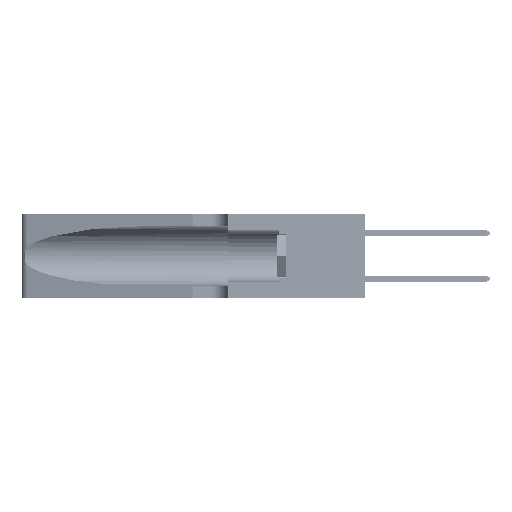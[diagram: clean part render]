
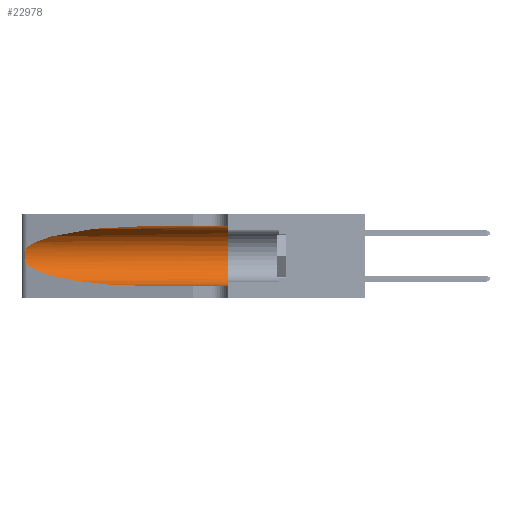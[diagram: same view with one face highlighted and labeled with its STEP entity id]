
A CAD part, left-side view. The second image highlights one B-rep face of the part: STEP entity #22978.
In plain terms, the highlighted cylindrical face has radius 3.308 mm (diameter 6.617 mm), a partial arc.
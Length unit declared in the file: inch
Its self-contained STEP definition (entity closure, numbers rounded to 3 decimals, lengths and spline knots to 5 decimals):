
#62 = CARTESIAN_POINT ( 'NONE',  ( 0.18966, 0.96281, 0.31525 ) ) ;
#373 =( BOUNDED_CURVE ( )  B_SPLINE_CURVE ( 3, ( #7837, #62, #42143, #19459 ),
 .UNSPECIFIED., .F., .F. ) 
 B_SPLINE_CURVE_WITH_KNOTS ( ( 4, 4 ),
 ( 1.5708, 2.84003 ),
 .UNSPECIFIED. ) 
 CURVE ( )  GEOMETRIC_REPRESENTATION_ITEM ( )  RATIONAL_B_SPLINE_CURVE ( ( 1., 0.87, 0.87, 1. ) ) 
 REPRESENTATION_ITEM ( '' )  );
#442 = ORIENTED_EDGE ( 'NONE', *, *, #43985, .F. ) ;
#2747 = CARTESIAN_POINT ( 'NONE',  ( 0.1305, 1.61858, 0.31525 ) ) ;
#2788 = CARTESIAN_POINT ( 'NONE',  ( 0.25487, 1.22718, 0.22369 ) ) ;
#5811 = ORIENTED_EDGE ( 'NONE', *, *, #29733, .F. ) ;
#6112 = DIRECTION ( 'NONE',  ( 0., 1., 0. ) ) ;
#6242 = VERTEX_POINT ( 'NONE', #46862 ) ;
#6470 = AXIS2_PLACEMENT_3D ( 'NONE', #29033, #6112, #32855 ) ;
#6654 = CARTESIAN_POINT ( 'NONE',  ( 0.25787, 1.23484, 0.2124 ) ) ;
#7378 = CYLINDRICAL_SURFACE ( 'NONE', #45912, 0.13025 ) ;
#7679 = LINE ( 'NONE', #2747, #47015 ) ;
#7837 = CARTESIAN_POINT ( 'NONE',  ( 0.1305, 0.72297, 0.31525 ) ) ;
#8088 = ORIENTED_EDGE ( 'NONE', *, *, #19232, .T. ) ;
#9329 = B_SPLINE_CURVE_WITH_KNOTS ( 'NONE', 3,
 ( #2788, #18099, #40841, #6654, #33392, #10520, #37198, #14399, #41004, #18273, #44805, #22125, #48634, #25943 ),
 .UNSPECIFIED., .F., .F.,
 ( 4, 2, 2, 2, 2, 2, 4 ),
 ( 0., 0.00027, 0.00053, 0.00107, 0.0016, 0.00187, 0.00214 ),
 .UNSPECIFIED. ) ;
#10520 = CARTESIAN_POINT ( 'NONE',  ( 0.26018, 1.23835, 0.19895 ) ) ;
#11185 = CARTESIAN_POINT ( 'NONE',  ( 0.18966, 0.96281, 0.05475 ) ) ;
#11971 = VERTEX_POINT ( 'NONE', #47407 ) ;
#13520 = ORIENTED_EDGE ( 'NONE', *, *, #34478, .T. ) ;
#14399 = CARTESIAN_POINT ( 'NONE',  ( 0.26075, 1.23896, 0.178 ) ) ;
#14514 = CARTESIAN_POINT ( 'NONE',  ( 0.25487, 1.22718, 0.14631 ) ) ;
#14601 =( BOUNDED_CURVE ( )  B_SPLINE_CURVE ( 3, ( #30231, #18780, #11185, #37859 ),
 .UNSPECIFIED., .F., .T. ) 
 B_SPLINE_CURVE_WITH_KNOTS ( ( 4, 4 ),
 ( 3.44316, 4.71239 ),
 .UNSPECIFIED. ) 
 CURVE ( )  GEOMETRIC_REPRESENTATION_ITEM ( )  RATIONAL_B_SPLINE_CURVE ( ( 1., 0.87, 0.87, 1. ) ) 
 REPRESENTATION_ITEM ( '' )  );
#16672 = CARTESIAN_POINT ( 'NONE',  ( 0.1305, 0.35, 0.31525 ) ) ;
#17841 = VERTEX_POINT ( 'NONE', #48037 ) ;
#18099 = CARTESIAN_POINT ( 'NONE',  ( 0.25555, 1.22994, 0.2215 ) ) ;
#18226 = DIRECTION ( 'NONE',  ( 0., -1., 0. ) ) ;
#18273 = CARTESIAN_POINT ( 'NONE',  ( 0.25856, 1.23593, 0.16098 ) ) ;
#18780 = CARTESIAN_POINT ( 'NONE',  ( 0.2373, 1.15595, 0.08982 ) ) ;
#19232 = EDGE_CURVE ( 'NONE', #17841, #11971, #25170, .T. ) ;
#19459 = CARTESIAN_POINT ( 'NONE',  ( 0.25487, 1.22718, 0.22369 ) ) ;
#21739 = CARTESIAN_POINT ( 'NONE',  ( 0.1305, 1.61858, 0.05475 ) ) ;
#22125 = CARTESIAN_POINT ( 'NONE',  ( 0.25639, 1.23186, 0.15144 ) ) ;
#22978 = ADVANCED_FACE ( 'NONE', ( #49098 ), #7378, .F. ) ;
#25170 = LINE ( 'NONE', #21739, #44121 ) ;
#25538 = DIRECTION ( 'NONE',  ( 0., -1., 0. ) ) ;
#25943 = CARTESIAN_POINT ( 'NONE',  ( 0.25487, 1.22718, 0.14631 ) ) ;
#29033 = CARTESIAN_POINT ( 'NONE',  ( 0.1305, 0.35, 0.185 ) ) ;
#29733 = EDGE_CURVE ( 'NONE', #42022, #11971, #30964, .T. ) ;
#30231 = CARTESIAN_POINT ( 'NONE',  ( 0.25487, 1.22718, 0.14631 ) ) ;
#30964 = CIRCLE ( 'NONE', #6470, 0.13025 ) ;
#31863 = CARTESIAN_POINT ( 'NONE',  ( 0.1305, 1.61858, 0.185 ) ) ;
#32312 = EDGE_CURVE ( 'NONE', #39011, #35049, #9329, .T. ) ;
#32855 = DIRECTION ( 'NONE',  ( 0., 0., 1. ) ) ;
#33392 = CARTESIAN_POINT ( 'NONE',  ( 0.25854, 1.2359, 0.20912 ) ) ;
#33879 = CARTESIAN_POINT ( 'NONE',  ( 0.25487, 1.22718, 0.22369 ) ) ;
#34478 = EDGE_CURVE ( 'NONE', #6242, #39011, #373, .T. ) ;
#35049 = VERTEX_POINT ( 'NONE', #14514 ) ;
#35666 = DIRECTION ( 'NONE',  ( 0., -1., 0. ) ) ;
#37198 = CARTESIAN_POINT ( 'NONE',  ( 0.26075, 1.23896, 0.19203 ) ) ;
#37328 = ORIENTED_EDGE ( 'NONE', *, *, #41092, .T. ) ;
#37859 = CARTESIAN_POINT ( 'NONE',  ( 0.1305, 0.72297, 0.05475 ) ) ;
#39011 = VERTEX_POINT ( 'NONE', #33879 ) ;
#40841 = CARTESIAN_POINT ( 'NONE',  ( 0.25639, 1.23184, 0.21858 ) ) ;
#41004 = CARTESIAN_POINT ( 'NONE',  ( 0.26017, 1.23833, 0.17102 ) ) ;
#41092 = EDGE_CURVE ( 'NONE', #35049, #17841, #14601, .T. ) ;
#42022 = VERTEX_POINT ( 'NONE', #16672 ) ;
#42143 = CARTESIAN_POINT ( 'NONE',  ( 0.2373, 1.15595, 0.28018 ) ) ;
#42753 = EDGE_LOOP ( 'NONE', ( #13520, #43825, #37328, #8088, #5811, #442 ) ) ;
#43136 = DIRECTION ( 'NONE',  ( 0., 0., -1. ) ) ;
#43825 = ORIENTED_EDGE ( 'NONE', *, *, #32312, .T. ) ;
#43985 = EDGE_CURVE ( 'NONE', #6242, #42022, #7679, .T. ) ;
#44121 = VECTOR ( 'NONE', #25538, 39.37008 ) ;
#44805 = CARTESIAN_POINT ( 'NONE',  ( 0.25789, 1.23486, 0.15765 ) ) ;
#45912 = AXIS2_PLACEMENT_3D ( 'NONE', #31863, #35666, #43136 ) ;
#46862 = CARTESIAN_POINT ( 'NONE',  ( 0.1305, 0.72297, 0.31525 ) ) ;
#47015 = VECTOR ( 'NONE', #18226, 39.37008 ) ;
#47407 = CARTESIAN_POINT ( 'NONE',  ( 0.1305, 0.35, 0.05475 ) ) ;
#48037 = CARTESIAN_POINT ( 'NONE',  ( 0.1305, 0.72297, 0.05475 ) ) ;
#48634 = CARTESIAN_POINT ( 'NONE',  ( 0.25555, 1.22993, 0.14849 ) ) ;
#49098 = FACE_OUTER_BOUND ( 'NONE', #42753, .T. ) ;
